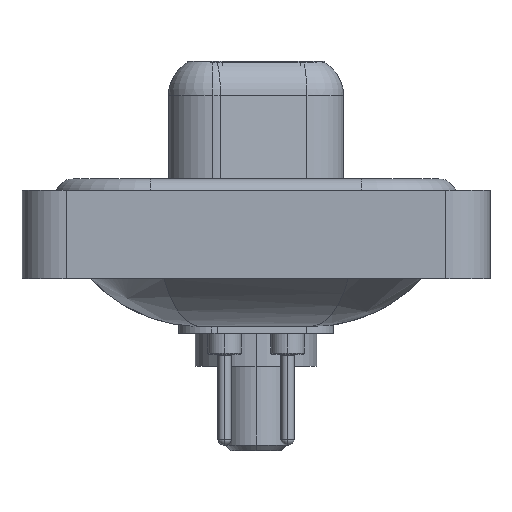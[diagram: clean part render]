
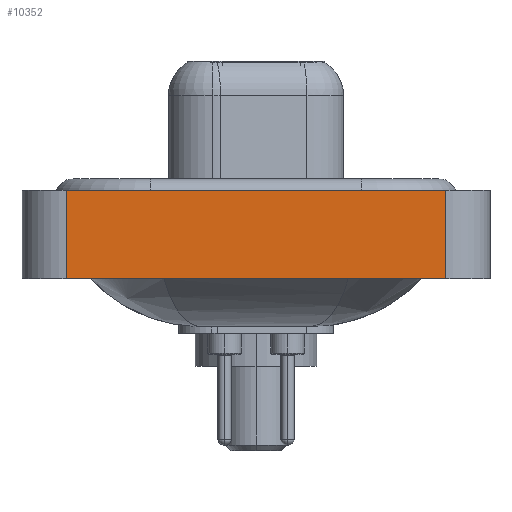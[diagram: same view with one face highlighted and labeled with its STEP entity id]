
A CAD part, left-side view. The second image highlights one B-rep face of the part: STEP entity #10352.
In plain terms, the highlighted planar face has unit normal (-1, 0, 0).
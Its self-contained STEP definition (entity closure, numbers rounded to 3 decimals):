
#1058 = CARTESIAN_POINT ( 'NONE',  ( -7.3, 8.55, -3.6 ) ) ;
#1904 = DIRECTION ( 'NONE',  ( 0., 0., 1. ) ) ;
#1919 = ORIENTED_EDGE ( 'NONE', *, *, #6310, .F. ) ;
#2050 = CARTESIAN_POINT ( 'NONE',  ( -7.3, -8.55, -3.6 ) ) ;
#3406 = CARTESIAN_POINT ( 'NONE',  ( -7.3, -8.55, 0.4 ) ) ;
#4311 = CARTESIAN_POINT ( 'NONE',  ( -7.3, -8.55, -3.6 ) ) ;
#4533 = LINE ( 'NONE', #4311, #17103 ) ;
#4798 = CARTESIAN_POINT ( 'NONE',  ( -7.3, 8.55, 0.4 ) ) ;
#4922 = CARTESIAN_POINT ( 'NONE',  ( -7.3, -8.55, 0.4 ) ) ;
#5344 = LINE ( 'NONE', #9042, #18569 ) ;
#5949 = EDGE_LOOP ( 'NONE', ( #15698, #10122, #1919, #18928 ) ) ;
#6212 = EDGE_CURVE ( 'NONE', #12256, #13376, #18441, .T. ) ;
#6310 = EDGE_CURVE ( 'NONE', #14795, #12256, #5344, .T. ) ;
#8664 = DIRECTION ( 'NONE',  ( -1., 0., 0. ) ) ;
#9042 = CARTESIAN_POINT ( 'NONE',  ( -7.3, 8.55, -3.6 ) ) ;
#9570 = DIRECTION ( 'NONE',  ( 0., -1., 0. ) ) ;
#10122 = ORIENTED_EDGE ( 'NONE', *, *, #6212, .F. ) ;
#10352 = ADVANCED_FACE ( 'NONE', ( #20688 ), #19136, .T. ) ;
#10440 = DIRECTION ( 'NONE',  ( 0., 0., 1. ) ) ;
#10648 = CARTESIAN_POINT ( 'NONE',  ( -7.3, -8.55, -3.6 ) ) ;
#11730 = DIRECTION ( 'NONE',  ( 0., -1., 0. ) ) ;
#12256 = VERTEX_POINT ( 'NONE', #4798 ) ;
#12311 = LINE ( 'NONE', #2050, #12672 ) ;
#12672 = VECTOR ( 'NONE', #17238, 1000. ) ;
#13376 = VERTEX_POINT ( 'NONE', #3406 ) ;
#14795 = VERTEX_POINT ( 'NONE', #1058 ) ;
#15698 = ORIENTED_EDGE ( 'NONE', *, *, #16282, .T. ) ;
#16282 = EDGE_CURVE ( 'NONE', #18122, #13376, #12311, .T. ) ;
#17103 = VECTOR ( 'NONE', #9570, 1000. ) ;
#17238 = DIRECTION ( 'NONE',  ( 0., 0., 1. ) ) ;
#17832 = CARTESIAN_POINT ( 'NONE',  ( -7.3, -8.55, -3.6 ) ) ;
#18122 = VERTEX_POINT ( 'NONE', #17832 ) ;
#18441 = LINE ( 'NONE', #4922, #20676 ) ;
#18569 = VECTOR ( 'NONE', #1904, 1000. ) ;
#18658 = AXIS2_PLACEMENT_3D ( 'NONE', #10648, #8664, #10440 ) ;
#18928 = ORIENTED_EDGE ( 'NONE', *, *, #19951, .T. ) ;
#19136 = PLANE ( 'NONE',  #18658 ) ;
#19951 = EDGE_CURVE ( 'NONE', #14795, #18122, #4533, .T. ) ;
#20676 = VECTOR ( 'NONE', #11730, 1000. ) ;
#20688 = FACE_OUTER_BOUND ( 'NONE', #5949, .T. ) ;
